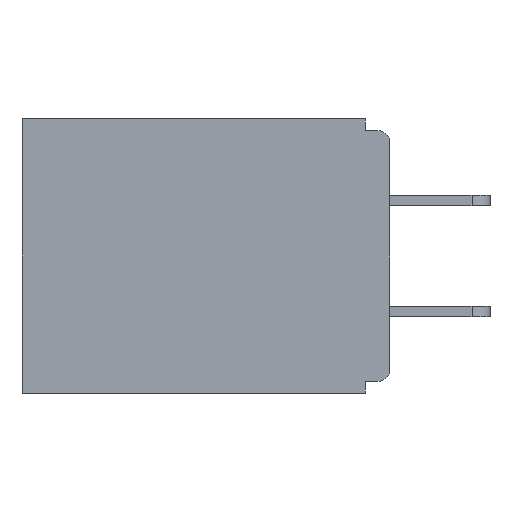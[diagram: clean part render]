
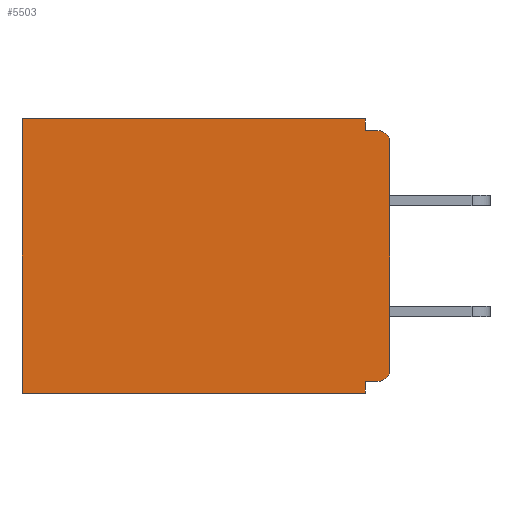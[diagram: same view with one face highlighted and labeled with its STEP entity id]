
A CAD part, left-side view. The second image highlights one B-rep face of the part: STEP entity #5503.
In plain terms, the highlighted planar face has unit normal (-1, 0, 0).
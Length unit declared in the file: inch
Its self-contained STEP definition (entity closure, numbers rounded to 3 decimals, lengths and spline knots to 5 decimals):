
#54 = EDGE_CURVE ( 'NONE', #7889, #13403, #13494, .T. ) ;
#67 = EDGE_CURVE ( 'NONE', #13403, #4807, #23524, .T. ) ;
#267 = EDGE_CURVE ( 'NONE', #24126, #17531, #12121, .T. ) ;
#318 = LINE ( 'NONE', #18884, #27502 ) ;
#432 = CARTESIAN_POINT ( 'NONE',  ( 0.298, 0.015, -0.03 ) ) ;
#522 = ORIENTED_EDGE ( 'NONE', *, *, #10968, .T. ) ;
#589 = VECTOR ( 'NONE', #19162, 39.37008 ) ;
#664 = DIRECTION ( 'NONE',  ( 0., 1., 0. ) ) ;
#1189 = DIRECTION ( 'NONE',  ( 0., 0., -1. ) ) ;
#1386 = CARTESIAN_POINT ( 'NONE',  ( 0.298, 0.46, 0. ) ) ;
#1929 = ORIENTED_EDGE ( 'NONE', *, *, #10484, .F. ) ;
#2106 = DIRECTION ( 'NONE',  ( 0., 0., -1. ) ) ;
#3817 = ORIENTED_EDGE ( 'NONE', *, *, #13322, .F. ) ;
#3868 = CARTESIAN_POINT ( 'NONE',  ( 0.298, 0., 0. ) ) ;
#4008 = ORIENTED_EDGE ( 'NONE', *, *, #6747, .F. ) ;
#4807 = VERTEX_POINT ( 'NONE', #9984 ) ;
#5409 = CARTESIAN_POINT ( 'NONE',  ( 0.298, 0., -0.313 ) ) ;
#5499 = ORIENTED_EDGE ( 'NONE', *, *, #17612, .F. ) ;
#5503 = ADVANCED_FACE ( 'NONE', ( #26158 ), #16734, .F. ) ;
#5748 = EDGE_CURVE ( 'NONE', #22121, #17531, #318, .T. ) ;
#6070 = DIRECTION ( 'NONE',  ( 0., 0., -1. ) ) ;
#6098 = CARTESIAN_POINT ( 'NONE',  ( 0.298, 0.031, -0.015 ) ) ;
#6257 = VECTOR ( 'NONE', #1189, 39.37008 ) ;
#6747 = EDGE_CURVE ( 'NONE', #21306, #4807, #18730, .T. ) ;
#6929 = CARTESIAN_POINT ( 'NONE',  ( 0.298, 0.015, -0.313 ) ) ;
#7609 = LINE ( 'NONE', #11662, #6257 ) ;
#7706 = VECTOR ( 'NONE', #19875, 39.37008 ) ;
#7879 = CARTESIAN_POINT ( 'NONE',  ( 0.298, 0., 0. ) ) ;
#7889 = VERTEX_POINT ( 'NONE', #23976 ) ;
#7987 = VERTEX_POINT ( 'NONE', #5409 ) ;
#8030 = DIRECTION ( 'NONE',  ( 0., -1., 0. ) ) ;
#8069 = CARTESIAN_POINT ( 'NONE',  ( 0.298, 0.46, 0. ) ) ;
#9119 = VECTOR ( 'NONE', #664, 39.37008 ) ;
#9797 = CIRCLE ( 'NONE', #17325, 0.015 ) ;
#9984 = CARTESIAN_POINT ( 'NONE',  ( 0.298, 0.46, -0.343 ) ) ;
#10081 = EDGE_CURVE ( 'NONE', #24126, #7987, #17206, .T. ) ;
#10484 = EDGE_CURVE ( 'NONE', #24440, #26945, #13167, .T. ) ;
#10968 = EDGE_CURVE ( 'NONE', #24440, #7987, #9797, .T. ) ;
#11062 = ORIENTED_EDGE ( 'NONE', *, *, #67, .T. ) ;
#11084 = LINE ( 'NONE', #11683, #7706 ) ;
#11264 = DIRECTION ( 'NONE',  ( -1., 0., 0. ) ) ;
#11391 = CARTESIAN_POINT ( 'NONE',  ( 0.298, 0., -0.328 ) ) ;
#11448 = ORIENTED_EDGE ( 'NONE', *, *, #5748, .F. ) ;
#11530 = VECTOR ( 'NONE', #6070, 39.37008 ) ;
#11662 = CARTESIAN_POINT ( 'NONE',  ( 0.298, 0.031, -0.343 ) ) ;
#11683 = CARTESIAN_POINT ( 'NONE',  ( 0.298, 0.031, -0.343 ) ) ;
#12118 = DIRECTION ( 'NONE',  ( 0., 1., 0. ) ) ;
#12121 = CIRCLE ( 'NONE', #27345, 0.015 ) ;
#12653 = CARTESIAN_POINT ( 'NONE',  ( 0.298, 0., 0. ) ) ;
#12944 = CARTESIAN_POINT ( 'NONE',  ( 0.298, 0.031, -0.328 ) ) ;
#13137 = CARTESIAN_POINT ( 'NONE',  ( 0.298, 0.015, -0.328 ) ) ;
#13167 = LINE ( 'NONE', #11391, #9119 ) ;
#13322 = EDGE_CURVE ( 'NONE', #7889, #22121, #7609, .T. ) ;
#13403 = VERTEX_POINT ( 'NONE', #8069 ) ;
#13494 = LINE ( 'NONE', #7879, #18501 ) ;
#15072 = DIRECTION ( 'NONE',  ( -1., 0., 0. ) ) ;
#15953 = EDGE_LOOP ( 'NONE', ( #17219, #11448, #3817, #22207, #11062, #4008, #5499, #1929, #522, #23720 ) ) ;
#16406 = DIRECTION ( 'NONE',  ( 0., 0., -1. ) ) ;
#16720 = CARTESIAN_POINT ( 'NONE',  ( 0.298, 0.031, -0.343 ) ) ;
#16734 = PLANE ( 'NONE',  #22811 ) ;
#17206 = LINE ( 'NONE', #12653, #11530 ) ;
#17208 = CARTESIAN_POINT ( 'NONE',  ( 0.298, 0., -0.343 ) ) ;
#17219 = ORIENTED_EDGE ( 'NONE', *, *, #267, .T. ) ;
#17325 = AXIS2_PLACEMENT_3D ( 'NONE', #6929, #11264, #26251 ) ;
#17531 = VERTEX_POINT ( 'NONE', #24026 ) ;
#17612 = EDGE_CURVE ( 'NONE', #26945, #21306, #11084, .T. ) ;
#17825 = VECTOR ( 'NONE', #16406, 39.37008 ) ;
#18501 = VECTOR ( 'NONE', #12118, 39.37008 ) ;
#18730 = LINE ( 'NONE', #17208, #589 ) ;
#18884 = CARTESIAN_POINT ( 'NONE',  ( 0.298, 0., -0.015 ) ) ;
#19162 = DIRECTION ( 'NONE',  ( 0., 1., 0. ) ) ;
#19875 = DIRECTION ( 'NONE',  ( 0., 0., -1. ) ) ;
#20571 = CARTESIAN_POINT ( 'NONE',  ( 0.298, 0., -0.03 ) ) ;
#21033 = DIRECTION ( 'NONE',  ( 1., 0., 0. ) ) ;
#21306 = VERTEX_POINT ( 'NONE', #16720 ) ;
#22121 = VERTEX_POINT ( 'NONE', #6098 ) ;
#22207 = ORIENTED_EDGE ( 'NONE', *, *, #54, .T. ) ;
#22811 = AXIS2_PLACEMENT_3D ( 'NONE', #3868, #21033, #23213 ) ;
#23213 = DIRECTION ( 'NONE',  ( 0., 0., -1. ) ) ;
#23524 = LINE ( 'NONE', #1386, #17825 ) ;
#23720 = ORIENTED_EDGE ( 'NONE', *, *, #10081, .F. ) ;
#23976 = CARTESIAN_POINT ( 'NONE',  ( 0.298, 0.031, 0. ) ) ;
#24026 = CARTESIAN_POINT ( 'NONE',  ( 0.298, 0.015, -0.015 ) ) ;
#24126 = VERTEX_POINT ( 'NONE', #20571 ) ;
#24440 = VERTEX_POINT ( 'NONE', #13137 ) ;
#26158 = FACE_OUTER_BOUND ( 'NONE', #15953, .T. ) ;
#26251 = DIRECTION ( 'NONE',  ( 0., 0., -1. ) ) ;
#26945 = VERTEX_POINT ( 'NONE', #12944 ) ;
#27345 = AXIS2_PLACEMENT_3D ( 'NONE', #432, #15072, #2106 ) ;
#27502 = VECTOR ( 'NONE', #8030, 39.37008 ) ;
